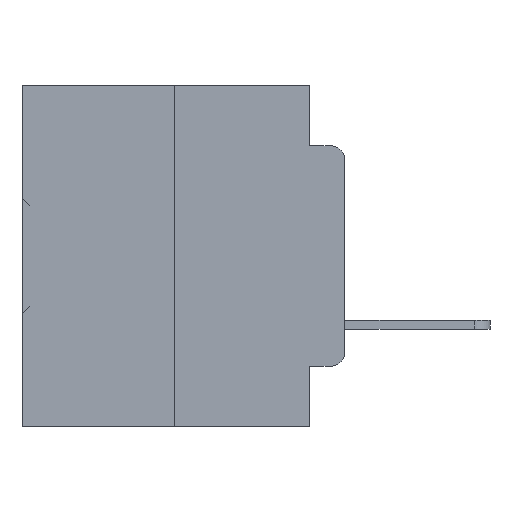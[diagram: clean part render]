
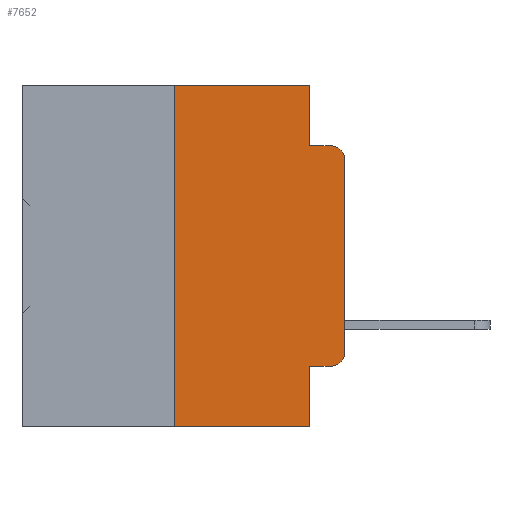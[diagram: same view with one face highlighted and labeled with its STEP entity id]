
A CAD part, left-side view. The second image highlights one B-rep face of the part: STEP entity #7652.
In plain terms, the highlighted planar face has unit normal (-1, 0, 0).
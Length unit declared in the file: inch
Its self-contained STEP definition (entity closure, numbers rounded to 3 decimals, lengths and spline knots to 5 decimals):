
#37 = CARTESIAN_POINT ( 'NONE',  ( 0., 0.02, -0.4115 ) ) ;
#211 = VECTOR ( 'NONE', #14443, 39.37008 ) ;
#611 = VERTEX_POINT ( 'NONE', #25311 ) ;
#679 = ORIENTED_EDGE ( 'NONE', *, *, #37679, .F. ) ;
#1695 = ORIENTED_EDGE ( 'NONE', *, *, #14278, .F. ) ;
#2181 = ORIENTED_EDGE ( 'NONE', *, *, #10562, .F. ) ;
#3155 = DIRECTION ( 'NONE',  ( 1., 0., 0. ) ) ;
#4751 = EDGE_CURVE ( 'NONE', #6475, #20826, #31347, .T. ) ;
#5159 = DIRECTION ( 'NONE',  ( 0., -1., 0. ) ) ;
#6196 = DIRECTION ( 'NONE',  ( -1., 0., 0. ) ) ;
#6217 = LINE ( 'NONE', #32858, #21501 ) ;
#6475 = VERTEX_POINT ( 'NONE', #37 ) ;
#6855 = ORIENTED_EDGE ( 'NONE', *, *, #32077, .T. ) ;
#7422 = CARTESIAN_POINT ( 'NONE',  ( 0., 0.25, 0. ) ) ;
#7652 = ADVANCED_FACE ( 'NONE', ( #10402 ), #12228, .F. ) ;
#10227 = ORIENTED_EDGE ( 'NONE', *, *, #37945, .F. ) ;
#10302 = CARTESIAN_POINT ( 'NONE',  ( 0., 0.051, 0. ) ) ;
#10402 = FACE_OUTER_BOUND ( 'NONE', #17258, .T. ) ;
#10562 = EDGE_CURVE ( 'NONE', #34694, #13321, #19048, .T. ) ;
#10725 = LINE ( 'NONE', #35177, #38452 ) ;
#11289 = CARTESIAN_POINT ( 'NONE',  ( 0., 0.02, -0.0885 ) ) ;
#11343 = CARTESIAN_POINT ( 'NONE',  ( 0., 0.051, -0.4115 ) ) ;
#11467 = EDGE_CURVE ( 'NONE', #13321, #30169, #27495, .T. ) ;
#12228 = PLANE ( 'NONE',  #17349 ) ;
#13321 = VERTEX_POINT ( 'NONE', #28382 ) ;
#13363 = DIRECTION ( 'NONE',  ( 0., 0., -1. ) ) ;
#14278 = EDGE_CURVE ( 'NONE', #31891, #611, #32285, .T. ) ;
#14443 = DIRECTION ( 'NONE',  ( 0., 0., -1. ) ) ;
#15010 = ORIENTED_EDGE ( 'NONE', *, *, #36977, .T. ) ;
#15065 = CARTESIAN_POINT ( 'NONE',  ( 0., 0.02, -0.1085 ) ) ;
#15564 = AXIS2_PLACEMENT_3D ( 'NONE', #15065, #35712, #18074 ) ;
#15847 = LINE ( 'NONE', #34472, #30825 ) ;
#16806 = EDGE_CURVE ( 'NONE', #22068, #38276, #36261, .T. ) ;
#17046 = DIRECTION ( 'NONE',  ( 0., -1., 0. ) ) ;
#17258 = EDGE_LOOP ( 'NONE', ( #15010, #23992, #679, #19743, #2181, #10227, #6855, #1695, #26883, #34521 ) ) ;
#17326 = CARTESIAN_POINT ( 'NONE',  ( 0., 0.25, -0.5 ) ) ;
#17349 = AXIS2_PLACEMENT_3D ( 'NONE', #21385, #3155, #24411 ) ;
#17985 = CARTESIAN_POINT ( 'NONE',  ( 0., 0.051, -0.0885 ) ) ;
#18074 = DIRECTION ( 'NONE',  ( 0., 0., -1. ) ) ;
#19048 = LINE ( 'NONE', #20080, #26148 ) ;
#19743 = ORIENTED_EDGE ( 'NONE', *, *, #11467, .F. ) ;
#20080 = CARTESIAN_POINT ( 'NONE',  ( 0., 0.473, 0. ) ) ;
#20531 = VECTOR ( 'NONE', #5159, 39.37008 ) ;
#20826 = VERTEX_POINT ( 'NONE', #29476 ) ;
#21385 = CARTESIAN_POINT ( 'NONE',  ( 0., 0.473, 0. ) ) ;
#21481 = LINE ( 'NONE', #11343, #20531 ) ;
#21501 = VECTOR ( 'NONE', #29989, 39.37008 ) ;
#22068 = VERTEX_POINT ( 'NONE', #35345 ) ;
#23992 = ORIENTED_EDGE ( 'NONE', *, *, #16806, .T. ) ;
#24411 = DIRECTION ( 'NONE',  ( 0., 0., -1. ) ) ;
#24453 = CARTESIAN_POINT ( 'NONE',  ( 0., 0.02, -0.3915 ) ) ;
#25311 = CARTESIAN_POINT ( 'NONE',  ( 0., 0.051, -0.5 ) ) ;
#25368 = VECTOR ( 'NONE', #34030, 39.37008 ) ;
#25667 = VECTOR ( 'NONE', #13363, 39.37008 ) ;
#26148 = VECTOR ( 'NONE', #17046, 39.37008 ) ;
#26883 = ORIENTED_EDGE ( 'NONE', *, *, #34877, .T. ) ;
#27138 = VERTEX_POINT ( 'NONE', #17326 ) ;
#27453 = DIRECTION ( 'NONE',  ( 0., 0., -1. ) ) ;
#27495 = LINE ( 'NONE', #10302, #25667 ) ;
#28382 = CARTESIAN_POINT ( 'NONE',  ( 0., 0.051, 0. ) ) ;
#29439 = CARTESIAN_POINT ( 'NONE',  ( 0., 0.051, 0. ) ) ;
#29476 = CARTESIAN_POINT ( 'NONE',  ( 0., 0., -0.3915 ) ) ;
#29989 = DIRECTION ( 'NONE',  ( 0., 0., 1. ) ) ;
#30169 = VERTEX_POINT ( 'NONE', #17985 ) ;
#30825 = VECTOR ( 'NONE', #37307, 39.37008 ) ;
#31200 = CARTESIAN_POINT ( 'NONE',  ( 0., 0., 0. ) ) ;
#31347 = CIRCLE ( 'NONE', #37852, 0.02 ) ;
#31891 = VERTEX_POINT ( 'NONE', #34191 ) ;
#32077 = EDGE_CURVE ( 'NONE', #27138, #611, #10725, .T. ) ;
#32285 = LINE ( 'NONE', #29439, #211 ) ;
#32858 = CARTESIAN_POINT ( 'NONE',  ( 0., 0.25, 0. ) ) ;
#33987 = LINE ( 'NONE', #31200, #25368 ) ;
#34030 = DIRECTION ( 'NONE',  ( 0., 0., 1. ) ) ;
#34191 = CARTESIAN_POINT ( 'NONE',  ( 0., 0.051, -0.4115 ) ) ;
#34472 = CARTESIAN_POINT ( 'NONE',  ( 0., 0.051, -0.0885 ) ) ;
#34521 = ORIENTED_EDGE ( 'NONE', *, *, #4751, .T. ) ;
#34694 = VERTEX_POINT ( 'NONE', #7422 ) ;
#34877 = EDGE_CURVE ( 'NONE', #31891, #6475, #21481, .T. ) ;
#35177 = CARTESIAN_POINT ( 'NONE',  ( 0., 0.473, -0.5 ) ) ;
#35345 = CARTESIAN_POINT ( 'NONE',  ( 0., 0., -0.1085 ) ) ;
#35712 = DIRECTION ( 'NONE',  ( -1., 0., 0. ) ) ;
#36261 = CIRCLE ( 'NONE', #15564, 0.02 ) ;
#36977 = EDGE_CURVE ( 'NONE', #20826, #22068, #33987, .T. ) ;
#37307 = DIRECTION ( 'NONE',  ( 0., -1., 0. ) ) ;
#37679 = EDGE_CURVE ( 'NONE', #30169, #38276, #15847, .T. ) ;
#37852 = AXIS2_PLACEMENT_3D ( 'NONE', #24453, #6196, #27453 ) ;
#37945 = EDGE_CURVE ( 'NONE', #27138, #34694, #6217, .T. ) ;
#37995 = DIRECTION ( 'NONE',  ( 0., -1., 0. ) ) ;
#38276 = VERTEX_POINT ( 'NONE', #11289 ) ;
#38452 = VECTOR ( 'NONE', #37995, 39.37008 ) ;
